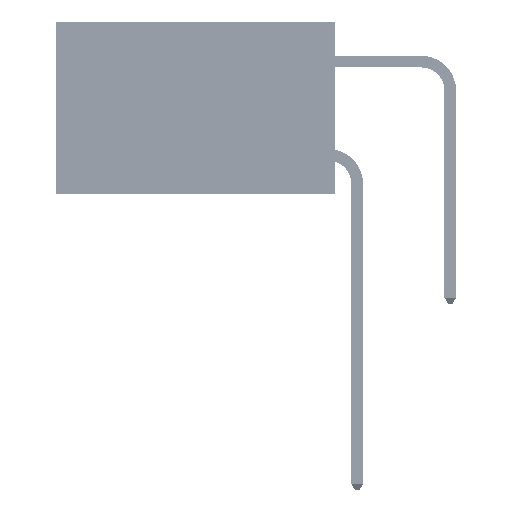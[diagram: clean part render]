
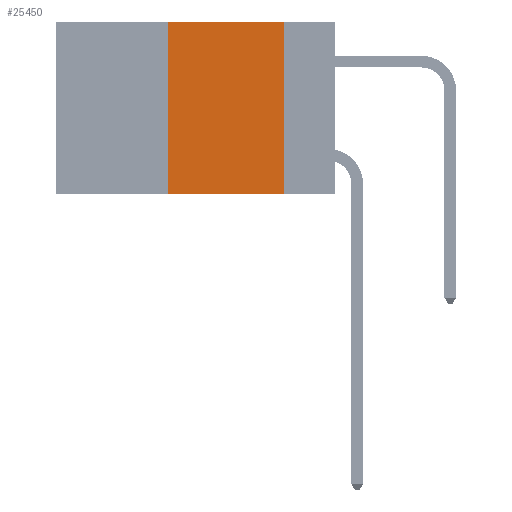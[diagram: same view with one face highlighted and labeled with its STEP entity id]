
A CAD part, left-side view. The second image highlights one B-rep face of the part: STEP entity #25450.
In plain terms, the highlighted planar face has unit normal (-1, 0, 0).
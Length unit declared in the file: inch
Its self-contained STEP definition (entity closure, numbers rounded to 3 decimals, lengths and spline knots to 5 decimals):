
#170 = CARTESIAN_POINT ( 'NONE',  ( 0., 0.36, 0. ) ) ;
#781 = EDGE_CURVE ( 'NONE', #28140, #5676, #24265, .T. ) ;
#3052 = DIRECTION ( 'NONE',  ( 0., -1., 0. ) ) ;
#3139 = DIRECTION ( 'NONE',  ( 0., 0., -1. ) ) ;
#5676 = VERTEX_POINT ( 'NONE', #170 ) ;
#6775 = CARTESIAN_POINT ( 'NONE',  ( 0., 0.36, 0. ) ) ;
#9842 = LINE ( 'NONE', #50078, #20270 ) ;
#10503 = FACE_OUTER_BOUND ( 'NONE', #15655, .T. ) ;
#12165 = CARTESIAN_POINT ( 'NONE',  ( 0., 0.11, 0. ) ) ;
#13755 = ORIENTED_EDGE ( 'NONE', *, *, #31905, .T. ) ;
#14042 = CARTESIAN_POINT ( 'NONE',  ( 0., 0.11, -0.37 ) ) ;
#15655 = EDGE_LOOP ( 'NONE', ( #29707, #20498, #22978, #13755 ) ) ;
#20270 = VECTOR ( 'NONE', #3052, 39.37008 ) ;
#20498 = ORIENTED_EDGE ( 'NONE', *, *, #37745, .F. ) ;
#21977 = CARTESIAN_POINT ( 'NONE',  ( 0., 0.36, -0.37 ) ) ;
#22899 = CARTESIAN_POINT ( 'NONE',  ( 0., 0.6, 0. ) ) ;
#22978 = ORIENTED_EDGE ( 'NONE', *, *, #781, .F. ) ;
#24265 = LINE ( 'NONE', #6775, #32225 ) ;
#24392 = EDGE_CURVE ( 'NONE', #27423, #45847, #29649, .T. ) ;
#25450 = ADVANCED_FACE ( 'NONE', ( #10503 ), #46258, .F. ) ;
#26837 = DIRECTION ( 'NONE',  ( 1., 0., 0. ) ) ;
#27423 = VERTEX_POINT ( 'NONE', #49020 ) ;
#28140 = VERTEX_POINT ( 'NONE', #21977 ) ;
#29649 = LINE ( 'NONE', #12165, #41245 ) ;
#29707 = ORIENTED_EDGE ( 'NONE', *, *, #24392, .F. ) ;
#30333 = DIRECTION ( 'NONE',  ( 0., 0., 1. ) ) ;
#31905 = EDGE_CURVE ( 'NONE', #28140, #45847, #9842, .T. ) ;
#32225 = VECTOR ( 'NONE', #30333, 39.37008 ) ;
#33674 = VECTOR ( 'NONE', #41822, 39.37008 ) ;
#36123 = LINE ( 'NONE', #49644, #33674 ) ;
#37745 = EDGE_CURVE ( 'NONE', #5676, #27423, #36123, .T. ) ;
#39551 = DIRECTION ( 'NONE',  ( 0., 0., -1. ) ) ;
#41245 = VECTOR ( 'NONE', #39551, 39.37008 ) ;
#41822 = DIRECTION ( 'NONE',  ( 0., -1., 0. ) ) ;
#45847 = VERTEX_POINT ( 'NONE', #14042 ) ;
#45864 = AXIS2_PLACEMENT_3D ( 'NONE', #22899, #26837, #3139 ) ;
#46258 = PLANE ( 'NONE',  #45864 ) ;
#49020 = CARTESIAN_POINT ( 'NONE',  ( 0., 0.11, 0. ) ) ;
#49644 = CARTESIAN_POINT ( 'NONE',  ( 0., 0.6, 0. ) ) ;
#50078 = CARTESIAN_POINT ( 'NONE',  ( 0., 0.6, -0.37 ) ) ;
